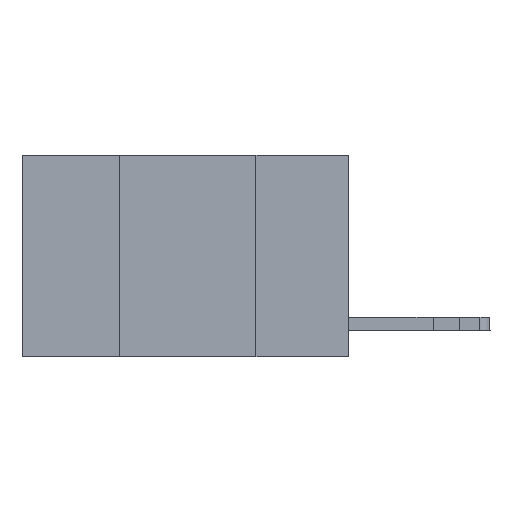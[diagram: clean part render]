
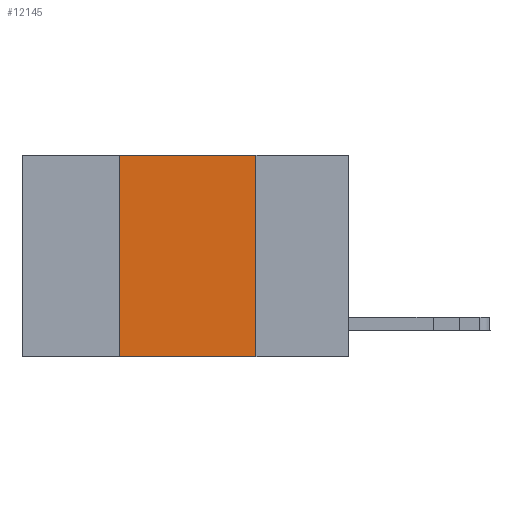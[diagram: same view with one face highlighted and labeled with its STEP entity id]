
A CAD part, left-side view. The second image highlights one B-rep face of the part: STEP entity #12145.
In plain terms, the highlighted planar face has unit normal (-1, 0, 0).
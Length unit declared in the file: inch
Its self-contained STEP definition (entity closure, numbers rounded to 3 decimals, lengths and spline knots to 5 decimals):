
#26 = EDGE_LOOP ( 'NONE', ( #14283, #15309, #11062, #3778 ) ) ;
#253 = VECTOR ( 'NONE', #14322, 39.37008 ) ;
#481 = CARTESIAN_POINT ( 'NONE',  ( 0., 0.6, -0.37 ) ) ;
#906 = AXIS2_PLACEMENT_3D ( 'NONE', #5003, #9894, #14710 ) ;
#1531 = LINE ( 'NONE', #2788, #253 ) ;
#1699 = DIRECTION ( 'NONE',  ( 0., 0., 1. ) ) ;
#1770 = VERTEX_POINT ( 'NONE', #3860 ) ;
#1838 = LINE ( 'NONE', #481, #2575 ) ;
#1921 = CARTESIAN_POINT ( 'NONE',  ( 0., 0.42, 0. ) ) ;
#2575 = VECTOR ( 'NONE', #12968, 39.37008 ) ;
#2788 = CARTESIAN_POINT ( 'NONE',  ( 0., 0.6, 0. ) ) ;
#3623 = EDGE_CURVE ( 'NONE', #7590, #4945, #5602, .T. ) ;
#3778 = ORIENTED_EDGE ( 'NONE', *, *, #7036, .T. ) ;
#3860 = CARTESIAN_POINT ( 'NONE',  ( 0., 0.17, -0.37 ) ) ;
#4328 = EDGE_CURVE ( 'NONE', #4945, #14096, #1531, .T. ) ;
#4923 = PLANE ( 'NONE',  #906 ) ;
#4945 = VERTEX_POINT ( 'NONE', #7331 ) ;
#5003 = CARTESIAN_POINT ( 'NONE',  ( 0., 0.6, 0. ) ) ;
#5602 = LINE ( 'NONE', #1921, #11339 ) ;
#6198 = CARTESIAN_POINT ( 'NONE',  ( 0., 0.42, -0.37 ) ) ;
#7036 = EDGE_CURVE ( 'NONE', #7590, #1770, #1838, .T. ) ;
#7331 = CARTESIAN_POINT ( 'NONE',  ( 0., 0.42, 0. ) ) ;
#7590 = VERTEX_POINT ( 'NONE', #6198 ) ;
#9813 = FACE_OUTER_BOUND ( 'NONE', #26, .T. ) ;
#9847 = CARTESIAN_POINT ( 'NONE',  ( 0., 0.17, 0. ) ) ;
#9894 = DIRECTION ( 'NONE',  ( 1., 0., 0. ) ) ;
#9983 = EDGE_CURVE ( 'NONE', #14096, #1770, #10874, .T. ) ;
#10874 = LINE ( 'NONE', #9847, #15182 ) ;
#11062 = ORIENTED_EDGE ( 'NONE', *, *, #3623, .F. ) ;
#11339 = VECTOR ( 'NONE', #1699, 39.37008 ) ;
#12145 = ADVANCED_FACE ( 'NONE', ( #9813 ), #4923, .F. ) ;
#12252 = CARTESIAN_POINT ( 'NONE',  ( 0., 0.17, 0. ) ) ;
#12403 = DIRECTION ( 'NONE',  ( 0., 0., -1. ) ) ;
#12968 = DIRECTION ( 'NONE',  ( 0., -1., 0. ) ) ;
#14096 = VERTEX_POINT ( 'NONE', #12252 ) ;
#14283 = ORIENTED_EDGE ( 'NONE', *, *, #9983, .F. ) ;
#14322 = DIRECTION ( 'NONE',  ( 0., -1., 0. ) ) ;
#14710 = DIRECTION ( 'NONE',  ( 0., 0., -1. ) ) ;
#15182 = VECTOR ( 'NONE', #12403, 39.37008 ) ;
#15309 = ORIENTED_EDGE ( 'NONE', *, *, #4328, .F. ) ;
